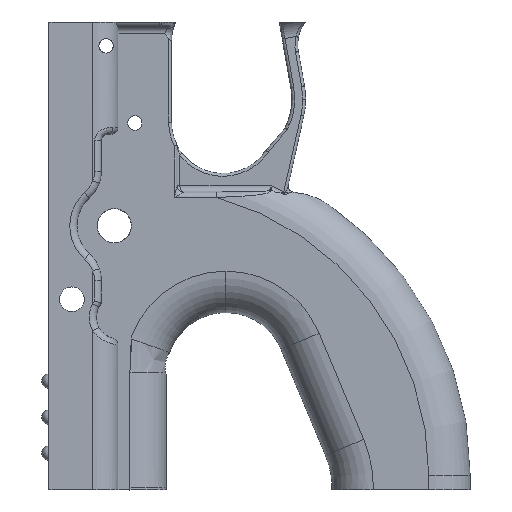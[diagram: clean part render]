
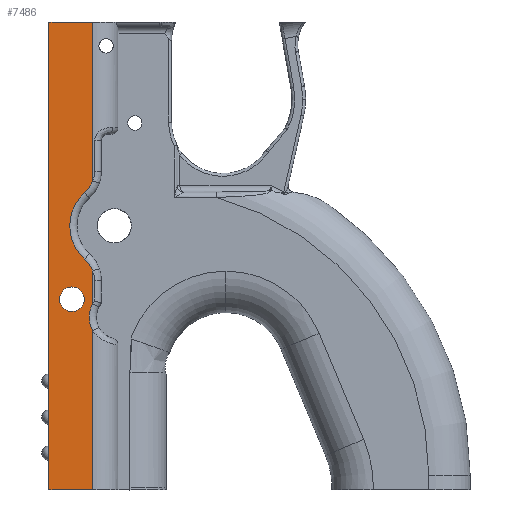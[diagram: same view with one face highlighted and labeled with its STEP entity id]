
A CAD part, left-side view. The second image highlights one B-rep face of the part: STEP entity #7486.
In plain terms, the highlighted planar face has unit normal (-1, 0, 0).
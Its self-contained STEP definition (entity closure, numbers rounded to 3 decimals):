
#141 = CIRCLE ( 'NONE', #8560, 3.429 ) ;
#148 = EDGE_CURVE ( 'NONE', #10225, #6332, #5967, .T. ) ;
#369 = CARTESIAN_POINT ( 'NONE',  ( 55.44, 32.37, 139.98 ) ) ;
#400 = DIRECTION ( 'NONE',  ( 0., 0., 1. ) ) ;
#562 = AXIS2_PLACEMENT_3D ( 'NONE', #6692, #3725, #3673 ) ;
#744 = DIRECTION ( 'NONE',  ( 0., 0., 1. ) ) ;
#900 = CARTESIAN_POINT ( 'NONE',  ( 55.44, 32.37, 139.98 ) ) ;
#1167 = CARTESIAN_POINT ( 'NONE',  ( 55.44, 32.37, 7.385 ) ) ;
#1177 = VECTOR ( 'NONE', #744, 1000. ) ;
#1196 = LINE ( 'NONE', #900, #1177 ) ;
#1383 = CARTESIAN_POINT ( 'NONE',  ( 55.44, 32.37, 32.527 ) ) ;
#1711 = ORIENTED_EDGE ( 'NONE', *, *, #10350, .T. ) ;
#1910 = CIRCLE ( 'NONE', #7742, 8. ) ;
#1959 = VERTEX_POINT ( 'NONE', #7176 ) ;
#1974 = DIRECTION ( 'NONE',  ( 0., 0., 1. ) ) ;
#1988 = CARTESIAN_POINT ( 'NONE',  ( 55.44, 32.37, 139.98 ) ) ;
#2047 = VERTEX_POINT ( 'NONE', #7650 ) ;
#2211 = CARTESIAN_POINT ( 'NONE',  ( 55.44, 39.935, 35.127 ) ) ;
#2475 = CARTESIAN_POINT ( 'NONE',  ( 55.44, 44.49, 76.582 ) ) ;
#2482 = DIRECTION ( 'NONE',  ( 0., 0., 1. ) ) ;
#2551 = CARTESIAN_POINT ( 'NONE',  ( 55.44, 34.6, 29.167 ) ) ;
#2714 = DIRECTION ( 'NONE',  ( -1., 0., 0. ) ) ;
#2765 = DIRECTION ( 'NONE',  ( 0., -1., 0. ) ) ;
#2784 = CARTESIAN_POINT ( 'NONE',  ( 55.44, 32.37, -1.656 ) ) ;
#3007 = EDGE_CURVE ( 'NONE', #4919, #3635, #1196, .T. ) ;
#3175 = DIRECTION ( 'NONE',  ( 0., 0., 1. ) ) ;
#3263 = DIRECTION ( 'NONE',  ( 0., 0., 1. ) ) ;
#3631 = CIRCLE ( 'NONE', #8922, 3.429 ) ;
#3635 = VERTEX_POINT ( 'NONE', #1167 ) ;
#3673 = DIRECTION ( 'NONE',  ( 0., 0., 1. ) ) ;
#3725 = DIRECTION ( 'NONE',  ( -1., 0., 0. ) ) ;
#3797 = EDGE_CURVE ( 'NONE', #12035, #2047, #141, .T. ) ;
#3800 = PLANE ( 'NONE',  #562 ) ;
#3974 = DIRECTION ( 'NONE',  ( 1., 0., 0. ) ) ;
#4377 = EDGE_CURVE ( 'NONE', #7785, #1959, #11795, .T. ) ;
#4548 = CIRCLE ( 'NONE', #11582, 12.362 ) ;
#4638 = LINE ( 'NONE', #7691, #4660 ) ;
#4660 = VECTOR ( 'NONE', #2765, 1000. ) ;
#4770 = EDGE_CURVE ( 'NONE', #3635, #6765, #11180, .T. ) ;
#4806 = EDGE_CURVE ( 'NONE', #7073, #6332, #11170, .T. ) ;
#4911 = VERTEX_POINT ( 'NONE', #2551 ) ;
#4919 = VERTEX_POINT ( 'NONE', #2784 ) ;
#5448 = CARTESIAN_POINT ( 'NONE',  ( 55.44, 38.127, -3.869 ) ) ;
#5601 = VERTEX_POINT ( 'NONE', #1383 ) ;
#5650 = ORIENTED_EDGE ( 'NONE', *, *, #4377, .T. ) ;
#5677 = ORIENTED_EDGE ( 'NONE', *, *, #148, .F. ) ;
#5821 = VECTOR ( 'NONE', #2482, 1000. ) ;
#5867 = DIRECTION ( 'NONE',  ( 0., 1., 0. ) ) ;
#5899 = CARTESIAN_POINT ( 'NONE',  ( 55.44, 32.37, 76.582 ) ) ;
#5967 = LINE ( 'NONE', #12273, #5821 ) ;
#6009 = CARTESIAN_POINT ( 'NONE',  ( 55.44, 39.935, 4.784 ) ) ;
#6170 = ORIENTED_EDGE ( 'NONE', *, *, #7698, .T. ) ;
#6205 = DIRECTION ( 'NONE',  ( 0., 0., 1. ) ) ;
#6243 = DIRECTION ( 'NONE',  ( 1., 0., 0. ) ) ;
#6285 = CARTESIAN_POINT ( 'NONE',  ( 55.44, 25.313, -5.444 ) ) ;
#6326 = CARTESIAN_POINT ( 'NONE',  ( 55.44, 32.37, 76.582 ) ) ;
#6332 = VERTEX_POINT ( 'NONE', #2475 ) ;
#6600 = ORIENTED_EDGE ( 'NONE', *, *, #10298, .T. ) ;
#6692 = CARTESIAN_POINT ( 'NONE',  ( 55.44, 32.37, 139.98 ) ) ;
#6763 = ORIENTED_EDGE ( 'NONE', *, *, #3797, .F. ) ;
#6765 = VERTEX_POINT ( 'NONE', #8555 ) ;
#6932 = ORIENTED_EDGE ( 'NONE', *, *, #3007, .T. ) ;
#7055 = EDGE_CURVE ( 'NONE', #5601, #7073, #8364, .T. ) ;
#7073 = VERTEX_POINT ( 'NONE', #6326 ) ;
#7099 = ORIENTED_EDGE ( 'NONE', *, *, #7055, .T. ) ;
#7176 = CARTESIAN_POINT ( 'NONE',  ( 55.44, 32.37, -9.232 ) ) ;
#7212 = AXIS2_PLACEMENT_3D ( 'NONE', #6009, #11532, #7510 ) ;
#7484 = CIRCLE ( 'NONE', #10201, 8.01 ) ;
#7486 = ADVANCED_FACE ( 'NONE', ( #7713, #7736 ), #3800, .T. ) ;
#7510 = DIRECTION ( 'NONE',  ( 0., 0., 1. ) ) ;
#7650 = CARTESIAN_POINT ( 'NONE',  ( 55.44, 38.127, 2.989 ) ) ;
#7691 = CARTESIAN_POINT ( 'NONE',  ( 55.44, 32.37, -53.418 ) ) ;
#7698 = EDGE_CURVE ( 'NONE', #1959, #4919, #7484, .T. ) ;
#7713 = FACE_BOUND ( 'NONE', #10187, .T. ) ;
#7736 = FACE_OUTER_BOUND ( 'NONE', #9695, .T. ) ;
#7742 = AXIS2_PLACEMENT_3D ( 'NONE', #2211, #8965, #3175 ) ;
#7785 = VERTEX_POINT ( 'NONE', #10631 ) ;
#8322 = CARTESIAN_POINT ( 'NONE',  ( 55.44, 38.127, -0.44 ) ) ;
#8364 = LINE ( 'NONE', #369, #8375 ) ;
#8375 = VECTOR ( 'NONE', #400, 1000. ) ;
#8518 = CARTESIAN_POINT ( 'NONE',  ( 55.44, 38.127, -0.44 ) ) ;
#8555 = CARTESIAN_POINT ( 'NONE',  ( 55.44, 34.6, 10.745 ) ) ;
#8560 = AXIS2_PLACEMENT_3D ( 'NONE', #8322, #10216, #3263 ) ;
#8922 = AXIS2_PLACEMENT_3D ( 'NONE', #8518, #2714, #9482 ) ;
#8965 = DIRECTION ( 'NONE',  ( -1., 0., 0. ) ) ;
#9001 = ORIENTED_EDGE ( 'NONE', *, *, #4770, .T. ) ;
#9482 = DIRECTION ( 'NONE',  ( 0., 0., 1. ) ) ;
#9612 = ORIENTED_EDGE ( 'NONE', *, *, #12325, .T. ) ;
#9695 = EDGE_LOOP ( 'NONE', ( #6932, #9001, #1711, #9612, #7099, #10092, #5677, #6600, #5650, #6170 ) ) ;
#9790 = CARTESIAN_POINT ( 'NONE',  ( 55.44, 26.354, 19.956 ) ) ;
#10092 = ORIENTED_EDGE ( 'NONE', *, *, #4806, .T. ) ;
#10187 = EDGE_LOOP ( 'NONE', ( #12341, #6763 ) ) ;
#10201 = AXIS2_PLACEMENT_3D ( 'NONE', #6285, #6243, #6205 ) ;
#10216 = DIRECTION ( 'NONE',  ( -1., 0., 0. ) ) ;
#10225 = VERTEX_POINT ( 'NONE', #12281 ) ;
#10298 = EDGE_CURVE ( 'NONE', #10225, #7785, #4638, .T. ) ;
#10350 = EDGE_CURVE ( 'NONE', #6765, #4911, #4548, .T. ) ;
#10631 = CARTESIAN_POINT ( 'NONE',  ( 55.44, 32.37, -53.418 ) ) ;
#10751 = DIRECTION ( 'NONE',  ( 0., 0., 1. ) ) ;
#11101 = VECTOR ( 'NONE', #5867, 1000. ) ;
#11170 = LINE ( 'NONE', #5899, #11101 ) ;
#11180 = CIRCLE ( 'NONE', #7212, 8. ) ;
#11265 = EDGE_CURVE ( 'NONE', #2047, #12035, #3631, .T. ) ;
#11532 = DIRECTION ( 'NONE',  ( -1., 0., 0. ) ) ;
#11582 = AXIS2_PLACEMENT_3D ( 'NONE', #9790, #3974, #10751 ) ;
#11728 = VECTOR ( 'NONE', #1974, 1000. ) ;
#11795 = LINE ( 'NONE', #1988, #11728 ) ;
#12035 = VERTEX_POINT ( 'NONE', #5448 ) ;
#12273 = CARTESIAN_POINT ( 'NONE',  ( 55.44, 44.49, 161.485 ) ) ;
#12281 = CARTESIAN_POINT ( 'NONE',  ( 55.44, 44.49, -53.418 ) ) ;
#12325 = EDGE_CURVE ( 'NONE', #4911, #5601, #1910, .T. ) ;
#12341 = ORIENTED_EDGE ( 'NONE', *, *, #11265, .F. ) ;
